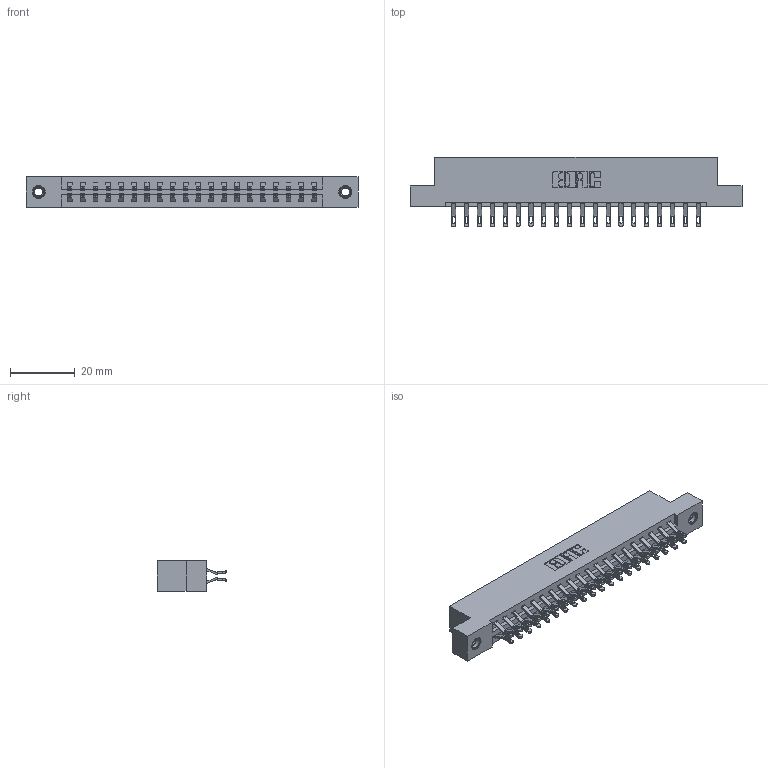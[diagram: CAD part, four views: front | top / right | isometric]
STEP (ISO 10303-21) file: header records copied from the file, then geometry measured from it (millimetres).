
FILE_DESCRIPTION (( 'STEP AP203' ), '1' );
FILE_NAME ('387-040-555-207.STEP', '2019-10-18T03:03:03', ( '' ), ( '' ), 'SwSTEP 2.0', 'SolidWorks 2016', '' );
FILE_SCHEMA (( 'CONFIG_CONTROL_DESIGN' ));
Length unit declared in the file: inch
Products named in the file (4): 387-040-555-207; 345-292-001_555 Tail; 337 Part_Flush Mounting Lugs - 0.156 Dia-TI; 345-250-001_345-250-005-103
Assembly tree (43 placements, depth 2):
  387-040-555-207
    337 Part_Flush Mounting Lugs - 0.156 Dia-TI
    345-292-001_555 Tail  x40
    345-250-001_345-250-005-103  x2
Bounding box: 102.26 x 21.47 x 9.4 mm (x, y, z)
Volume: 10586.7 mm3; surface area: 12227.7 mm2
Topology: 43 solids, 43 shells, 2574 faces, 8007 edges, 5330 vertices
Faces by surface type: plane 1542, cylinder 1016, cone 12, torus 4
Entity records: 19864 total; most frequent: CARTESIAN_POINT 3379, ORIENTED_EDGE 3278, DIRECTION 2917, EDGE_CURVE 1639, LINE 1471, VECTOR 1471, VERTEX_POINT 1088, AXIS2_PLACEMENT_3D 723
